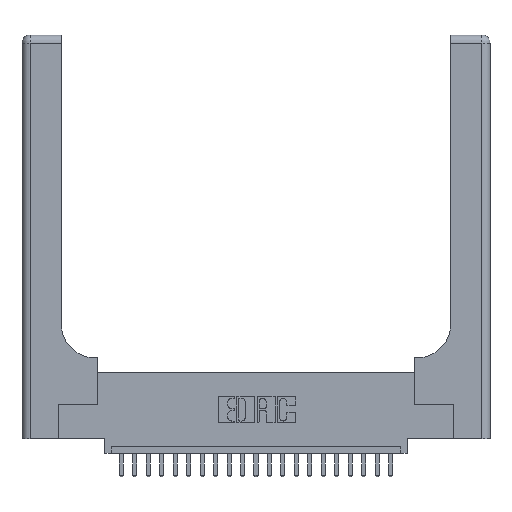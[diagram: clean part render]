
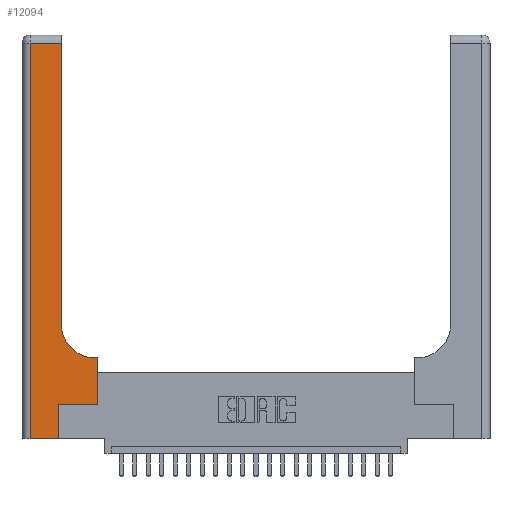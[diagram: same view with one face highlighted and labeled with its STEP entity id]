
A CAD part, top view. The second image highlights one B-rep face of the part: STEP entity #12094.
In plain terms, the highlighted planar face has unit normal (0, 0, 1).
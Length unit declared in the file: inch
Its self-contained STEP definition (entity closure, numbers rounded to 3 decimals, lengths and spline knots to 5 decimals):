
#416 = VERTEX_POINT ( 'NONE', #17507 ) ;
#640 = EDGE_CURVE ( 'NONE', #8912, #4753, #873, .T. ) ;
#873 = LINE ( 'NONE', #21562, #7294 ) ;
#1117 = EDGE_CURVE ( 'NONE', #18012, #17053, #11027, .T. ) ;
#1182 = CARTESIAN_POINT ( 'NONE',  ( 0.5415, 0.6, 0.37 ) ) ;
#1262 = CARTESIAN_POINT ( 'NONE',  ( 0.269, 0., 0.37 ) ) ;
#1713 = CARTESIAN_POINT ( 'NONE',  ( 0., 3., 0.37 ) ) ;
#2064 = AXIS2_PLACEMENT_3D ( 'NONE', #12659, #16378, #22064 ) ;
#2434 = CARTESIAN_POINT ( 'NONE',  ( 0., 2.94, 0.37 ) ) ;
#4409 = VECTOR ( 'NONE', #6024, 39.37008 ) ;
#4753 = VERTEX_POINT ( 'NONE', #1182 ) ;
#4908 = DIRECTION ( 'NONE',  ( 0., 1., 0. ) ) ;
#6024 = DIRECTION ( 'NONE',  ( -1., 0., 0. ) ) ;
#6323 = EDGE_LOOP ( 'NONE', ( #18332, #20430, #12693, #10237, #11485, #17490, #16204, #21784, #13581 ) ) ;
#6604 = VECTOR ( 'NONE', #15389, 39.37008 ) ;
#7077 = AXIS2_PLACEMENT_3D ( 'NONE', #1713, #9031, #20302 ) ;
#7294 = VECTOR ( 'NONE', #21474, 39.37008 ) ;
#7524 = FACE_OUTER_BOUND ( 'NONE', #6323, .T. ) ;
#7972 = CARTESIAN_POINT ( 'NONE',  ( 0.2915, 2.94, 0.37 ) ) ;
#8189 = LINE ( 'NONE', #2434, #4409 ) ;
#8532 = LINE ( 'NONE', #14517, #19169 ) ;
#8718 = CARTESIAN_POINT ( 'NONE',  ( 0.2915, 3., 0.37 ) ) ;
#8912 = VERTEX_POINT ( 'NONE', #22811 ) ;
#8946 = LINE ( 'NONE', #10800, #17640 ) ;
#9031 = DIRECTION ( 'NONE',  ( 0., 0., -1. ) ) ;
#9147 = EDGE_CURVE ( 'NONE', #17053, #13745, #8189, .T. ) ;
#9148 = VERTEX_POINT ( 'NONE', #20945 ) ;
#9709 = DIRECTION ( 'NONE',  ( 1., 0., 0. ) ) ;
#10022 = LINE ( 'NONE', #18962, #17271 ) ;
#10237 = ORIENTED_EDGE ( 'NONE', *, *, #14004, .T. ) ;
#10391 = CARTESIAN_POINT ( 'NONE',  ( 0.269, 0., 0.37 ) ) ;
#10800 = CARTESIAN_POINT ( 'NONE',  ( 0.06, 3., 0.37 ) ) ;
#11027 = LINE ( 'NONE', #8718, #14485 ) ;
#11485 = ORIENTED_EDGE ( 'NONE', *, *, #20814, .T. ) ;
#12094 = ADVANCED_FACE ( 'NONE', ( #7524 ), #14603, .F. ) ;
#12096 = VERTEX_POINT ( 'NONE', #1262 ) ;
#12207 = CIRCLE ( 'NONE', #2064, 0.25 ) ;
#12659 = CARTESIAN_POINT ( 'NONE',  ( 0.5415, 0.85, 0.37 ) ) ;
#12660 = DIRECTION ( 'NONE',  ( 0., -1., 0. ) ) ;
#12693 = ORIENTED_EDGE ( 'NONE', *, *, #20993, .T. ) ;
#12698 = LINE ( 'NONE', #15473, #6604 ) ;
#13092 = EDGE_CURVE ( 'NONE', #18683, #8912, #12698, .T. ) ;
#13202 = CARTESIAN_POINT ( 'NONE',  ( 0.2915, 0.85, 0.37 ) ) ;
#13581 = ORIENTED_EDGE ( 'NONE', *, *, #23511, .T. ) ;
#13745 = VERTEX_POINT ( 'NONE', #23856 ) ;
#14004 = EDGE_CURVE ( 'NONE', #416, #12096, #10022, .T. ) ;
#14485 = VECTOR ( 'NONE', #4908, 39.37008 ) ;
#14517 = CARTESIAN_POINT ( 'NONE',  ( 0.269, 0.25, 0.37 ) ) ;
#14603 = PLANE ( 'NONE',  #7077 ) ;
#15389 = DIRECTION ( 'NONE',  ( 0., 1., 0. ) ) ;
#15473 = CARTESIAN_POINT ( 'NONE',  ( 0.5585, 0.25, 0.37 ) ) ;
#15974 = DIRECTION ( 'NONE',  ( 0., 1., 0. ) ) ;
#16204 = ORIENTED_EDGE ( 'NONE', *, *, #13092, .T. ) ;
#16378 = DIRECTION ( 'NONE',  ( 0., 0., -1. ) ) ;
#17053 = VERTEX_POINT ( 'NONE', #7972 ) ;
#17271 = VECTOR ( 'NONE', #9709, 39.37008 ) ;
#17490 = ORIENTED_EDGE ( 'NONE', *, *, #23418, .T. ) ;
#17507 = CARTESIAN_POINT ( 'NONE',  ( 0.06, 0., 0.37 ) ) ;
#17640 = VECTOR ( 'NONE', #12660, 39.37008 ) ;
#17946 = VECTOR ( 'NONE', #15974, 39.37008 ) ;
#18012 = VERTEX_POINT ( 'NONE', #13202 ) ;
#18332 = ORIENTED_EDGE ( 'NONE', *, *, #1117, .T. ) ;
#18522 = DIRECTION ( 'NONE',  ( 1., 0., 0. ) ) ;
#18539 = LINE ( 'NONE', #10391, #17946 ) ;
#18683 = VERTEX_POINT ( 'NONE', #18935 ) ;
#18935 = CARTESIAN_POINT ( 'NONE',  ( 0.5585, 0.25, 0.37 ) ) ;
#18962 = CARTESIAN_POINT ( 'NONE',  ( 0., 0., 0.37 ) ) ;
#19169 = VECTOR ( 'NONE', #18522, 39.37008 ) ;
#20302 = DIRECTION ( 'NONE',  ( -1., 0., 0. ) ) ;
#20430 = ORIENTED_EDGE ( 'NONE', *, *, #9147, .T. ) ;
#20814 = EDGE_CURVE ( 'NONE', #12096, #9148, #18539, .T. ) ;
#20945 = CARTESIAN_POINT ( 'NONE',  ( 0.269, 0.25, 0.37 ) ) ;
#20993 = EDGE_CURVE ( 'NONE', #13745, #416, #8946, .T. ) ;
#21474 = DIRECTION ( 'NONE',  ( -1., 0., 0. ) ) ;
#21562 = CARTESIAN_POINT ( 'NONE',  ( 0.2915, 0.6, 0.37 ) ) ;
#21784 = ORIENTED_EDGE ( 'NONE', *, *, #640, .T. ) ;
#22064 = DIRECTION ( 'NONE',  ( 1., 0., 0. ) ) ;
#22811 = CARTESIAN_POINT ( 'NONE',  ( 0.5585, 0.6, 0.37 ) ) ;
#23418 = EDGE_CURVE ( 'NONE', #9148, #18683, #8532, .T. ) ;
#23511 = EDGE_CURVE ( 'NONE', #4753, #18012, #12207, .T. ) ;
#23856 = CARTESIAN_POINT ( 'NONE',  ( 0.06, 2.94, 0.37 ) ) ;
